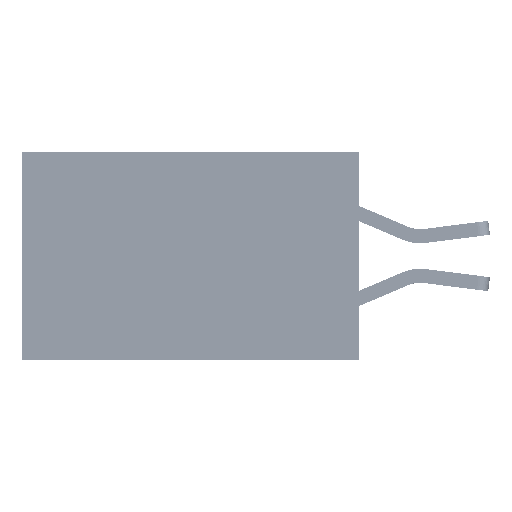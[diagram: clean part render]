
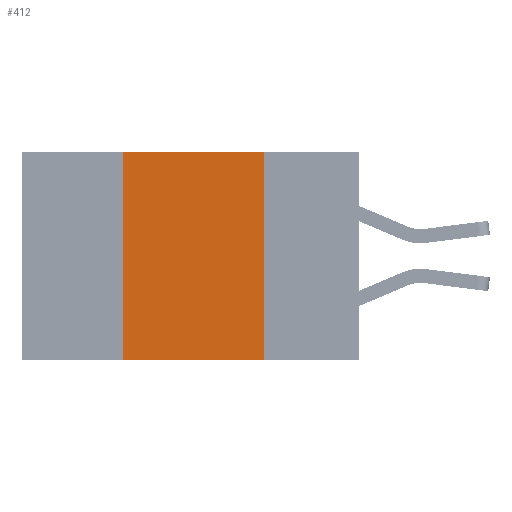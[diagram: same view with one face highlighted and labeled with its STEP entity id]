
A CAD part, left-side view. The second image highlights one B-rep face of the part: STEP entity #412.
In plain terms, the highlighted planar face has unit normal (-1, 0, 0).
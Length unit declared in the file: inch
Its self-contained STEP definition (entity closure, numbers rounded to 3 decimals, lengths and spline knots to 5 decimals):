
#238 = DIRECTION ( 'NONE',  ( 0., -1., 0. ) ) ;
#412 = ADVANCED_FACE ( 'NONE', ( #1496 ), #17675, .F. ) ;
#1496 = FACE_OUTER_BOUND ( 'NONE', #5640, .T. ) ;
#1513 = ORIENTED_EDGE ( 'NONE', *, *, #38462, .F. ) ;
#1698 = CARTESIAN_POINT ( 'NONE',  ( 0., 0.42, -0.37 ) ) ;
#3004 = VECTOR ( 'NONE', #238, 39.37008 ) ;
#5640 = EDGE_LOOP ( 'NONE', ( #1513, #13943, #42274, #38648 ) ) ;
#6060 = CARTESIAN_POINT ( 'NONE',  ( 0., 0.17, 0. ) ) ;
#10042 = VERTEX_POINT ( 'NONE', #12664 ) ;
#11321 = CARTESIAN_POINT ( 'NONE',  ( 0., 0.6, -0.37 ) ) ;
#12664 = CARTESIAN_POINT ( 'NONE',  ( 0., 0.17, 0. ) ) ;
#13943 = ORIENTED_EDGE ( 'NONE', *, *, #19589, .F. ) ;
#16972 = CARTESIAN_POINT ( 'NONE',  ( 0., 0.42, 0. ) ) ;
#17675 = PLANE ( 'NONE',  #47877 ) ;
#18591 = DIRECTION ( 'NONE',  ( 0., 0., 1. ) ) ;
#19390 = VECTOR ( 'NONE', #42793, 39.37008 ) ;
#19589 = EDGE_CURVE ( 'NONE', #49032, #10042, #41222, .T. ) ;
#19943 = CARTESIAN_POINT ( 'NONE',  ( 0., 0.6, 0. ) ) ;
#21643 = DIRECTION ( 'NONE',  ( 0., 0., -1. ) ) ;
#23218 = VECTOR ( 'NONE', #49257, 39.37008 ) ;
#28552 = VERTEX_POINT ( 'NONE', #1698 ) ;
#29422 = CARTESIAN_POINT ( 'NONE',  ( 0., 0.6, 0. ) ) ;
#29575 = VECTOR ( 'NONE', #18591, 39.37008 ) ;
#29897 = LINE ( 'NONE', #11321, #19390 ) ;
#33707 = LINE ( 'NONE', #6060, #23218 ) ;
#35661 = CARTESIAN_POINT ( 'NONE',  ( 0., 0.17, -0.37 ) ) ;
#38462 = EDGE_CURVE ( 'NONE', #10042, #46131, #33707, .T. ) ;
#38648 = ORIENTED_EDGE ( 'NONE', *, *, #39444, .T. ) ;
#39444 = EDGE_CURVE ( 'NONE', #28552, #46131, #29897, .T. ) ;
#41222 = LINE ( 'NONE', #19943, #3004 ) ;
#42179 = CARTESIAN_POINT ( 'NONE',  ( 0., 0.42, 0. ) ) ;
#42274 = ORIENTED_EDGE ( 'NONE', *, *, #50759, .F. ) ;
#42793 = DIRECTION ( 'NONE',  ( 0., -1., 0. ) ) ;
#45141 = DIRECTION ( 'NONE',  ( 1., 0., 0. ) ) ;
#46131 = VERTEX_POINT ( 'NONE', #35661 ) ;
#47877 = AXIS2_PLACEMENT_3D ( 'NONE', #29422, #45141, #21643 ) ;
#49032 = VERTEX_POINT ( 'NONE', #16972 ) ;
#49095 = LINE ( 'NONE', #42179, #29575 ) ;
#49257 = DIRECTION ( 'NONE',  ( 0., 0., -1. ) ) ;
#50759 = EDGE_CURVE ( 'NONE', #28552, #49032, #49095, .T. ) ;
